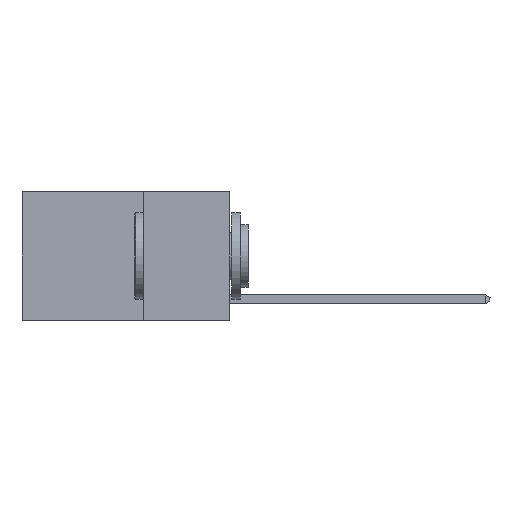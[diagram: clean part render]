
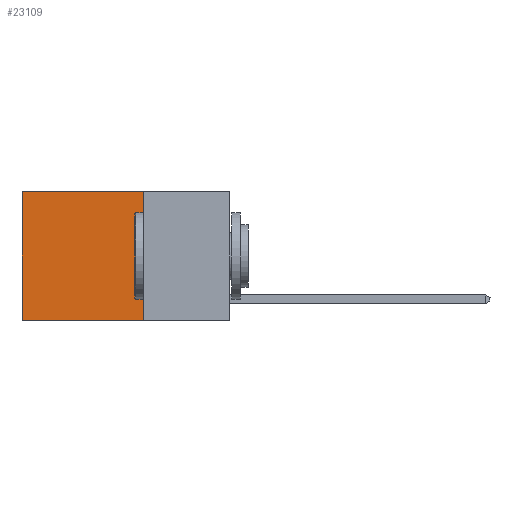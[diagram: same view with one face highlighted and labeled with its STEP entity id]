
A CAD part, left-side view. The second image highlights one B-rep face of the part: STEP entity #23109.
In plain terms, the highlighted planar face has unit normal (-1, 0, 0).
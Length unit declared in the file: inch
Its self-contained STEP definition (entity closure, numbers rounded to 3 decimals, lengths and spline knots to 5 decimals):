
#466 = VECTOR ( 'NONE', #12189, 39.37008 ) ;
#726 = VERTEX_POINT ( 'NONE', #18281 ) ;
#1489 = ORIENTED_EDGE ( 'NONE', *, *, #2810, .T. ) ;
#2058 = VECTOR ( 'NONE', #24731, 39.37008 ) ;
#2195 = CARTESIAN_POINT ( 'NONE',  ( 0.2625, 0.25, 0. ) ) ;
#2295 = PLANE ( 'NONE',  #9996 ) ;
#2810 = EDGE_CURVE ( 'NONE', #726, #12059, #15729, .T. ) ;
#3312 = EDGE_CURVE ( 'NONE', #726, #9804, #11793, .T. ) ;
#3924 = FACE_OUTER_BOUND ( 'NONE', #19067, .T. ) ;
#4408 = DIRECTION ( 'NONE',  ( 1., 0., 0. ) ) ;
#4679 = CARTESIAN_POINT ( 'NONE',  ( 0.2625, 0.25, -0.37 ) ) ;
#5678 = ORIENTED_EDGE ( 'NONE', *, *, #10655, .F. ) ;
#6201 = DIRECTION ( 'NONE',  ( 0., 0., -1. ) ) ;
#6566 = CARTESIAN_POINT ( 'NONE',  ( 0.2625, 0.6, -0.37 ) ) ;
#7074 = VERTEX_POINT ( 'NONE', #6566 ) ;
#7898 = CARTESIAN_POINT ( 'NONE',  ( 0.2625, 0.6, 0. ) ) ;
#9804 = VERTEX_POINT ( 'NONE', #17873 ) ;
#9811 = CARTESIAN_POINT ( 'NONE',  ( 0.2625, 0.6, 0. ) ) ;
#9996 = AXIS2_PLACEMENT_3D ( 'NONE', #23093, #4408, #21485 ) ;
#10655 = EDGE_CURVE ( 'NONE', #9804, #7074, #15985, .T. ) ;
#11758 = EDGE_CURVE ( 'NONE', #12059, #7074, #14914, .T. ) ;
#11793 = LINE ( 'NONE', #2195, #12750 ) ;
#12059 = VERTEX_POINT ( 'NONE', #7898 ) ;
#12189 = DIRECTION ( 'NONE',  ( 0., 1., 0. ) ) ;
#12750 = VECTOR ( 'NONE', #6201, 39.37008 ) ;
#14914 = LINE ( 'NONE', #9811, #18953 ) ;
#15729 = LINE ( 'NONE', #17136, #2058 ) ;
#15985 = LINE ( 'NONE', #4679, #466 ) ;
#17136 = CARTESIAN_POINT ( 'NONE',  ( 0.2625, 0.25, 0. ) ) ;
#17462 = DIRECTION ( 'NONE',  ( 0., 0., -1. ) ) ;
#17873 = CARTESIAN_POINT ( 'NONE',  ( 0.2625, 0.25, -0.37 ) ) ;
#18281 = CARTESIAN_POINT ( 'NONE',  ( 0.2625, 0.25, 0. ) ) ;
#18953 = VECTOR ( 'NONE', #17462, 39.37008 ) ;
#19067 = EDGE_LOOP ( 'NONE', ( #22492, #5678, #24595, #1489 ) ) ;
#21485 = DIRECTION ( 'NONE',  ( 0., 0., -1. ) ) ;
#22492 = ORIENTED_EDGE ( 'NONE', *, *, #11758, .T. ) ;
#23093 = CARTESIAN_POINT ( 'NONE',  ( 0.2625, 0.25, 0. ) ) ;
#23109 = ADVANCED_FACE ( 'NONE', ( #3924 ), #2295, .F. ) ;
#24595 = ORIENTED_EDGE ( 'NONE', *, *, #3312, .F. ) ;
#24731 = DIRECTION ( 'NONE',  ( 0., 1., 0. ) ) ;
